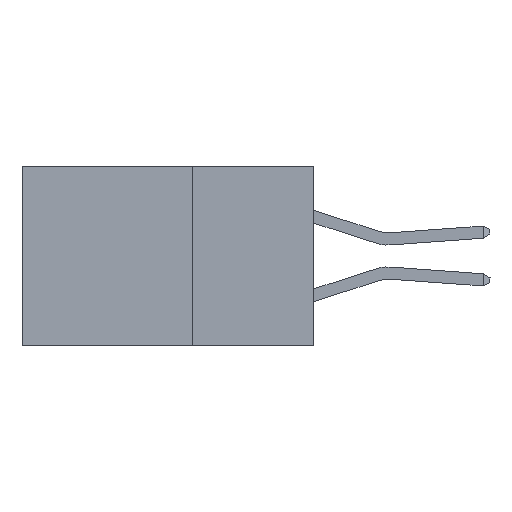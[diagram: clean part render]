
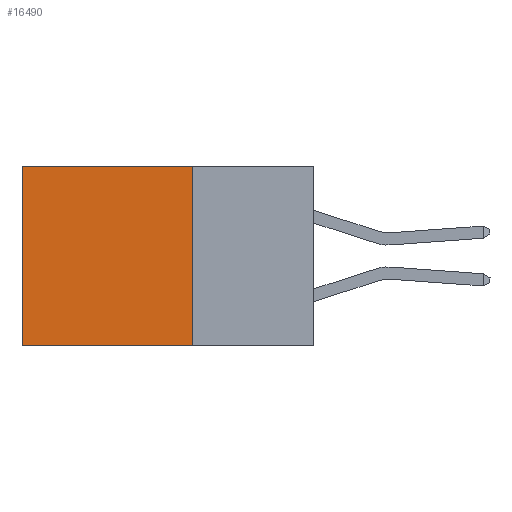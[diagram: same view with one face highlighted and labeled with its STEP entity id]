
A CAD part, left-side view. The second image highlights one B-rep face of the part: STEP entity #16490.
In plain terms, the highlighted planar face has unit normal (-1, 0, 0).
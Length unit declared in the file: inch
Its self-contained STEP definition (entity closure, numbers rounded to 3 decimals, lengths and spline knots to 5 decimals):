
#783 = AXIS2_PLACEMENT_3D ( 'NONE', #2071, #10453, #17598 ) ;
#1297 = DIRECTION ( 'NONE',  ( 0., 1., 0. ) ) ;
#1899 = CARTESIAN_POINT ( 'NONE',  ( 0.2875, 0.25, 0. ) ) ;
#2071 = CARTESIAN_POINT ( 'NONE',  ( 0.2875, 0.25, 0. ) ) ;
#2218 = VECTOR ( 'NONE', #11292, 39.37008 ) ;
#2459 = EDGE_CURVE ( 'NONE', #16563, #6507, #12320, .T. ) ;
#2697 = ORIENTED_EDGE ( 'NONE', *, *, #15535, .T. ) ;
#3463 = LINE ( 'NONE', #13545, #18058 ) ;
#3893 = EDGE_CURVE ( 'NONE', #15163, #6924, #15134, .T. ) ;
#4052 = ORIENTED_EDGE ( 'NONE', *, *, #2459, .T. ) ;
#4247 = FACE_OUTER_BOUND ( 'NONE', #11192, .T. ) ;
#5291 = CARTESIAN_POINT ( 'NONE',  ( 0.2875, 0.6, 0. ) ) ;
#5393 = LINE ( 'NONE', #15036, #13018 ) ;
#5482 = CARTESIAN_POINT ( 'NONE',  ( 0.2875, 0.6, -0.37 ) ) ;
#6507 = VERTEX_POINT ( 'NONE', #5482 ) ;
#6924 = VERTEX_POINT ( 'NONE', #8169 ) ;
#8169 = CARTESIAN_POINT ( 'NONE',  ( 0.2875, 0.25, -0.37 ) ) ;
#9830 = CARTESIAN_POINT ( 'NONE',  ( 0.2875, 0.6, 0. ) ) ;
#10429 = EDGE_CURVE ( 'NONE', #6924, #6507, #3463, .T. ) ;
#10453 = DIRECTION ( 'NONE',  ( 1., 0., 0. ) ) ;
#10811 = ORIENTED_EDGE ( 'NONE', *, *, #10429, .F. ) ;
#11192 = EDGE_LOOP ( 'NONE', ( #4052, #10811, #14029, #2697 ) ) ;
#11292 = DIRECTION ( 'NONE',  ( 0., 0., -1. ) ) ;
#12320 = LINE ( 'NONE', #9830, #13847 ) ;
#13018 = VECTOR ( 'NONE', #17807, 39.37008 ) ;
#13545 = CARTESIAN_POINT ( 'NONE',  ( 0.2875, 0.25, -0.37 ) ) ;
#13847 = VECTOR ( 'NONE', #13958, 39.37008 ) ;
#13952 = CARTESIAN_POINT ( 'NONE',  ( 0.2875, 0.25, 0. ) ) ;
#13958 = DIRECTION ( 'NONE',  ( 0., 0., -1. ) ) ;
#14029 = ORIENTED_EDGE ( 'NONE', *, *, #3893, .F. ) ;
#14742 = PLANE ( 'NONE',  #783 ) ;
#15036 = CARTESIAN_POINT ( 'NONE',  ( 0.2875, 0.25, 0. ) ) ;
#15134 = LINE ( 'NONE', #13952, #2218 ) ;
#15163 = VERTEX_POINT ( 'NONE', #1899 ) ;
#15535 = EDGE_CURVE ( 'NONE', #15163, #16563, #5393, .T. ) ;
#16490 = ADVANCED_FACE ( 'NONE', ( #4247 ), #14742, .F. ) ;
#16563 = VERTEX_POINT ( 'NONE', #5291 ) ;
#17598 = DIRECTION ( 'NONE',  ( 0., 0., -1. ) ) ;
#17807 = DIRECTION ( 'NONE',  ( 0., 1., 0. ) ) ;
#18058 = VECTOR ( 'NONE', #1297, 39.37008 ) ;
